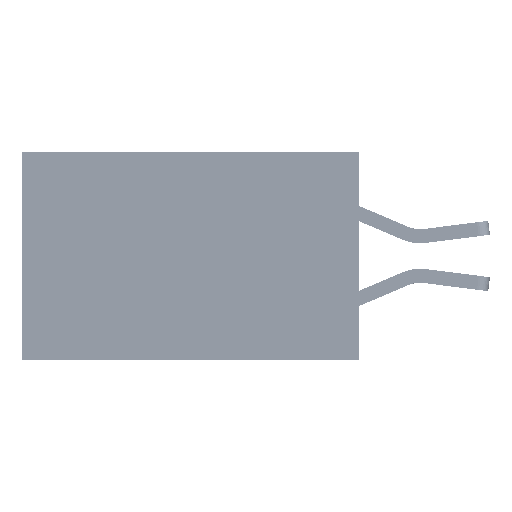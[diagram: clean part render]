
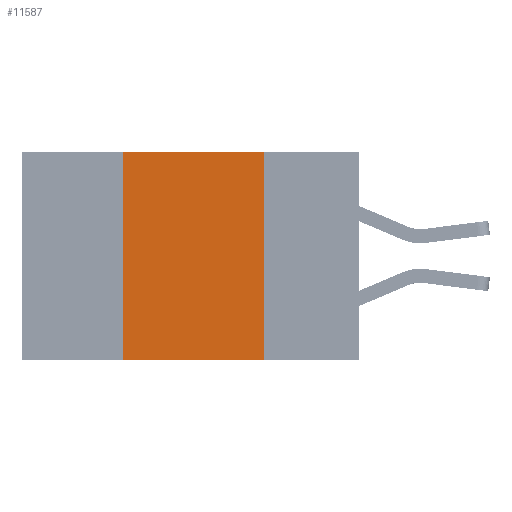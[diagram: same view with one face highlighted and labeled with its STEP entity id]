
A CAD part, left-side view. The second image highlights one B-rep face of the part: STEP entity #11587.
In plain terms, the highlighted planar face has unit normal (-1, 0, 0).
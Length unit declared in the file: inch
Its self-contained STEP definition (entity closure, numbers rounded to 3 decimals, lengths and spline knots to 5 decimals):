
#1142 = ORIENTED_EDGE ( 'NONE', *, *, #2274, .F. ) ;
#1342 = EDGE_LOOP ( 'NONE', ( #1142, #12279, #1343, #40620 ) ) ;
#1343 = ORIENTED_EDGE ( 'NONE', *, *, #38104, .F. ) ;
#1638 = CARTESIAN_POINT ( 'NONE',  ( 0., 0.42, -0.37 ) ) ;
#2274 = EDGE_CURVE ( 'NONE', #23504, #26566, #17732, .T. ) ;
#2514 = FACE_OUTER_BOUND ( 'NONE', #1342, .T. ) ;
#4068 = CARTESIAN_POINT ( 'NONE',  ( 0., 0.42, 0. ) ) ;
#6317 = EDGE_CURVE ( 'NONE', #11778, #26566, #25802, .T. ) ;
#6812 = CARTESIAN_POINT ( 'NONE',  ( 0., 0.6, -0.37 ) ) ;
#7820 = DIRECTION ( 'NONE',  ( 0., 0., -1. ) ) ;
#11587 = ADVANCED_FACE ( 'NONE', ( #2514 ), #15377, .F. ) ;
#11778 = VERTEX_POINT ( 'NONE', #1638 ) ;
#12279 = ORIENTED_EDGE ( 'NONE', *, *, #17723, .F. ) ;
#12531 = DIRECTION ( 'NONE',  ( 0., -1., 0. ) ) ;
#12850 = CARTESIAN_POINT ( 'NONE',  ( 0., 0.42, 0. ) ) ;
#14749 = CARTESIAN_POINT ( 'NONE',  ( 0., 0.6, 0. ) ) ;
#15377 = PLANE ( 'NONE',  #37209 ) ;
#17723 = EDGE_CURVE ( 'NONE', #27919, #23504, #18687, .T. ) ;
#17732 = LINE ( 'NONE', #40290, #40857 ) ;
#18331 = DIRECTION ( 'NONE',  ( 0., 0., -1. ) ) ;
#18687 = LINE ( 'NONE', #41464, #26776 ) ;
#21848 = DIRECTION ( 'NONE',  ( 0., -1., 0. ) ) ;
#23050 = DIRECTION ( 'NONE',  ( 0., 0., 1. ) ) ;
#23504 = VERTEX_POINT ( 'NONE', #25910 ) ;
#23665 = VECTOR ( 'NONE', #12531, 39.37008 ) ;
#25802 = LINE ( 'NONE', #6812, #23665 ) ;
#25910 = CARTESIAN_POINT ( 'NONE',  ( 0., 0.17, 0. ) ) ;
#26566 = VERTEX_POINT ( 'NONE', #28689 ) ;
#26776 = VECTOR ( 'NONE', #21848, 39.37008 ) ;
#27919 = VERTEX_POINT ( 'NONE', #12850 ) ;
#28362 = LINE ( 'NONE', #4068, #39035 ) ;
#28689 = CARTESIAN_POINT ( 'NONE',  ( 0., 0.17, -0.37 ) ) ;
#33933 = DIRECTION ( 'NONE',  ( 1., 0., 0. ) ) ;
#37209 = AXIS2_PLACEMENT_3D ( 'NONE', #14749, #33933, #18331 ) ;
#38104 = EDGE_CURVE ( 'NONE', #11778, #27919, #28362, .T. ) ;
#39035 = VECTOR ( 'NONE', #23050, 39.37008 ) ;
#40290 = CARTESIAN_POINT ( 'NONE',  ( 0., 0.17, 0. ) ) ;
#40620 = ORIENTED_EDGE ( 'NONE', *, *, #6317, .T. ) ;
#40857 = VECTOR ( 'NONE', #7820, 39.37008 ) ;
#41464 = CARTESIAN_POINT ( 'NONE',  ( 0., 0.6, 0. ) ) ;
